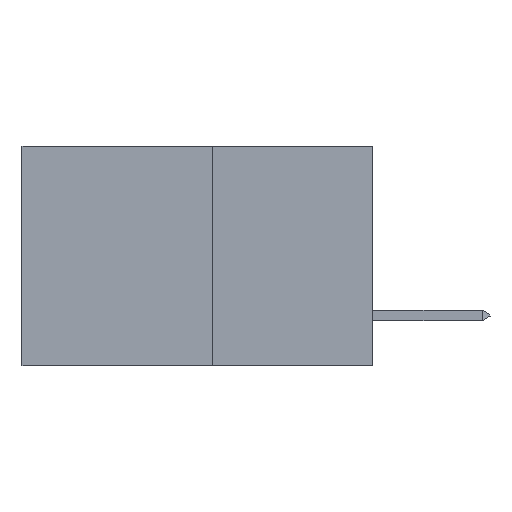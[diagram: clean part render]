
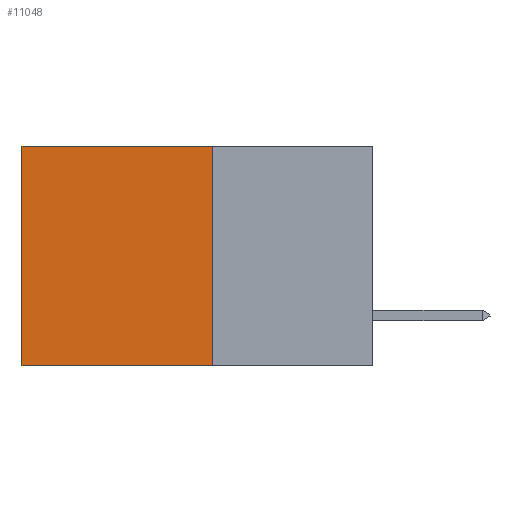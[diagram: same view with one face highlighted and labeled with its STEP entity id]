
A CAD part, left-side view. The second image highlights one B-rep face of the part: STEP entity #11048.
In plain terms, the highlighted planar face has unit normal (-1, 0, 0).
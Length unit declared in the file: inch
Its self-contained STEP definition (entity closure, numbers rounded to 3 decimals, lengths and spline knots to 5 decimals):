
#433 = EDGE_CURVE ( 'NONE', #3463, #7463, #3607, .T. ) ;
#1279 = VERTEX_POINT ( 'NONE', #4210 ) ;
#1459 = EDGE_LOOP ( 'NONE', ( #1791, #3462, #2882, #3200 ) ) ;
#1791 = ORIENTED_EDGE ( 'NONE', *, *, #2756, .T. ) ;
#2082 = VECTOR ( 'NONE', #8068, 39.37008 ) ;
#2281 = CARTESIAN_POINT ( 'NONE',  ( 0.277, 0.27, 0. ) ) ;
#2538 = CARTESIAN_POINT ( 'NONE',  ( 0.277, 0.27, -0.37 ) ) ;
#2662 = CARTESIAN_POINT ( 'NONE',  ( 0.277, 0.59, 0. ) ) ;
#2756 = EDGE_CURVE ( 'NONE', #7463, #3026, #4462, .T. ) ;
#2882 = ORIENTED_EDGE ( 'NONE', *, *, #5579, .F. ) ;
#3026 = VERTEX_POINT ( 'NONE', #3383 ) ;
#3200 = ORIENTED_EDGE ( 'NONE', *, *, #433, .T. ) ;
#3383 = CARTESIAN_POINT ( 'NONE',  ( 0.277, 0.59, -0.37 ) ) ;
#3462 = ORIENTED_EDGE ( 'NONE', *, *, #11531, .F. ) ;
#3463 = VERTEX_POINT ( 'NONE', #2281 ) ;
#3607 = LINE ( 'NONE', #3729, #6187 ) ;
#3729 = CARTESIAN_POINT ( 'NONE',  ( 0.277, 0.27, 0. ) ) ;
#4135 = CARTESIAN_POINT ( 'NONE',  ( 0.277, 0.27, -0.37 ) ) ;
#4210 = CARTESIAN_POINT ( 'NONE',  ( 0.277, 0.27, -0.37 ) ) ;
#4462 = LINE ( 'NONE', #8984, #2082 ) ;
#5127 = DIRECTION ( 'NONE',  ( 0., 0., -1. ) ) ;
#5232 = LINE ( 'NONE', #10713, #9763 ) ;
#5497 = VECTOR ( 'NONE', #10961, 39.37008 ) ;
#5579 = EDGE_CURVE ( 'NONE', #3463, #1279, #12440, .T. ) ;
#6187 = VECTOR ( 'NONE', #11812, 39.37008 ) ;
#7463 = VERTEX_POINT ( 'NONE', #2662 ) ;
#8068 = DIRECTION ( 'NONE',  ( 0., 0., -1. ) ) ;
#8957 = PLANE ( 'NONE',  #11662 ) ;
#8984 = CARTESIAN_POINT ( 'NONE',  ( 0.277, 0.59, -0.37 ) ) ;
#9763 = VECTOR ( 'NONE', #11633, 39.37008 ) ;
#10713 = CARTESIAN_POINT ( 'NONE',  ( 0.277, 0.27, -0.37 ) ) ;
#10859 = DIRECTION ( 'NONE',  ( 1., 0., 0. ) ) ;
#10961 = DIRECTION ( 'NONE',  ( 0., 0., -1. ) ) ;
#11048 = ADVANCED_FACE ( 'NONE', ( #12174 ), #8957, .F. ) ;
#11531 = EDGE_CURVE ( 'NONE', #1279, #3026, #5232, .T. ) ;
#11633 = DIRECTION ( 'NONE',  ( 0., 1., 0. ) ) ;
#11662 = AXIS2_PLACEMENT_3D ( 'NONE', #4135, #10859, #5127 ) ;
#11812 = DIRECTION ( 'NONE',  ( 0., 1., 0. ) ) ;
#12174 = FACE_OUTER_BOUND ( 'NONE', #1459, .T. ) ;
#12440 = LINE ( 'NONE', #2538, #5497 ) ;
